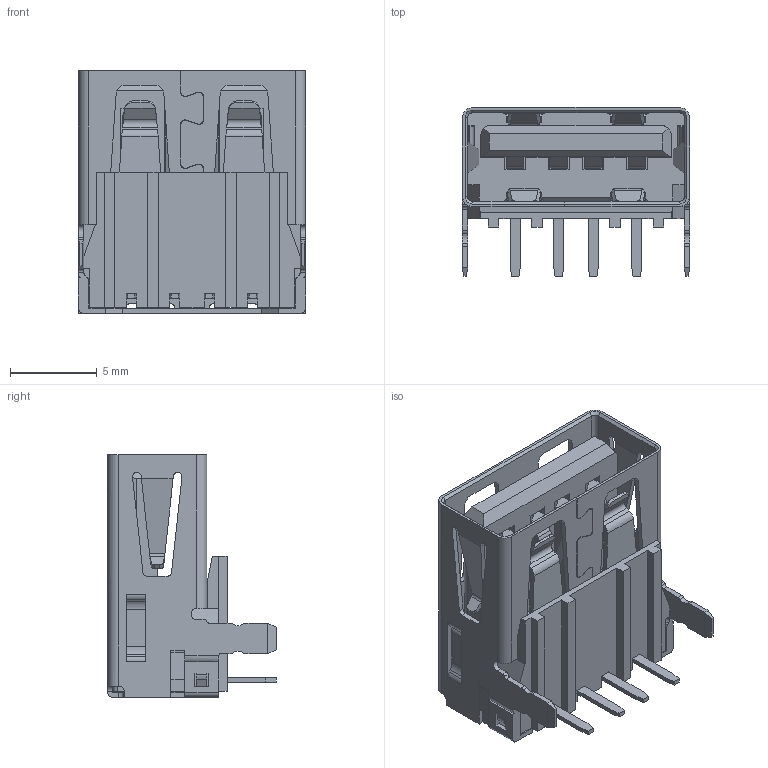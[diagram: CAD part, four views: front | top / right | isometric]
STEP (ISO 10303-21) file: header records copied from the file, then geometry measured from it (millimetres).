
FILE_DESCRIPTION (( 'STEP AP214' ), '1' );
FILE_NAME ('690A104-621-241.STEP', '2021-01-13T21:06:26', ( '' ), ( '' ), 'SwSTEP 2.0', 'SolidWorks 2020', '' );
FILE_SCHEMA (( 'AUTOMOTIVE_DESIGN' ));
Length unit declared in the file: millimetre
Products named in the file (4): Shell 690A104-621-241; Contact 690A104-621-241; Insulator 690A104-621-241; 690A104-621-241
Assembly tree (6 placements, depth 2):
  690A104-621-241
    Insulator 690A104-621-241
    Contact 690A104-621-241  x4
    Shell 690A104-621-241
Bounding box: 13.1 x 9.73 x 14 mm (x, y, z)
Volume: 566.5 mm3; surface area: 2082.6 mm2
Topology: 6 solids, 6 shells, 929 faces, 2638 edges, 1700 vertices
Faces by surface type: plane 632, cylinder 201, bspline 92, cone 4
Entity records: 27993 total; most frequent: CARTESIAN_POINT 8861, ORIENTED_EDGE 4268, DIRECTION 3488, EDGE_CURVE 2134, LINE 1576, VECTOR 1576, VERTEX_POINT 1364, AXIS2_PLACEMENT_3D 956
